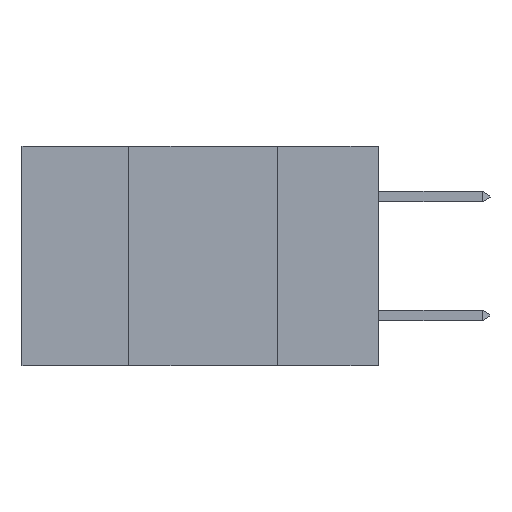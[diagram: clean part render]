
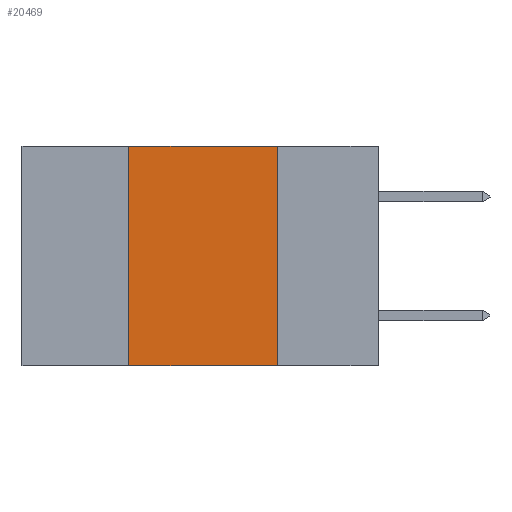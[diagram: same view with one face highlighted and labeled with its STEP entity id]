
A CAD part, left-side view. The second image highlights one B-rep face of the part: STEP entity #20469.
In plain terms, the highlighted planar face has unit normal (-1, 0, 0).
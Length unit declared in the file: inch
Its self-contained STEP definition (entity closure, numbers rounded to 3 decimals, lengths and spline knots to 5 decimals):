
#223 = CARTESIAN_POINT ( 'NONE',  ( 0., 0.6, -0.37 ) ) ;
#341 = DIRECTION ( 'NONE',  ( 0., 0., 1. ) ) ;
#450 = EDGE_CURVE ( 'NONE', #16474, #4178, #8391, .T. ) ;
#529 = ORIENTED_EDGE ( 'NONE', *, *, #15107, .F. ) ;
#792 = VERTEX_POINT ( 'NONE', #21328 ) ;
#1607 = CARTESIAN_POINT ( 'NONE',  ( 0., 0.6, 0. ) ) ;
#2045 = CARTESIAN_POINT ( 'NONE',  ( 0., 0.42, 0. ) ) ;
#2080 = LINE ( 'NONE', #223, #2353 ) ;
#2353 = VECTOR ( 'NONE', #6689, 39.37008 ) ;
#4178 = VERTEX_POINT ( 'NONE', #13958 ) ;
#5643 = VECTOR ( 'NONE', #8329, 39.37008 ) ;
#6024 = VECTOR ( 'NONE', #9877, 39.37008 ) ;
#6689 = DIRECTION ( 'NONE',  ( 0., -1., 0. ) ) ;
#8209 = ORIENTED_EDGE ( 'NONE', *, *, #450, .F. ) ;
#8329 = DIRECTION ( 'NONE',  ( 0., -1., 0. ) ) ;
#8335 = DIRECTION ( 'NONE',  ( 0., 0., -1. ) ) ;
#8364 = ORIENTED_EDGE ( 'NONE', *, *, #14026, .T. ) ;
#8391 = LINE ( 'NONE', #2045, #12371 ) ;
#8765 = FACE_OUTER_BOUND ( 'NONE', #16736, .T. ) ;
#8934 = LINE ( 'NONE', #11384, #6024 ) ;
#9877 = DIRECTION ( 'NONE',  ( 0., 0., -1. ) ) ;
#10109 = CARTESIAN_POINT ( 'NONE',  ( 0., 0.6, 0. ) ) ;
#11384 = CARTESIAN_POINT ( 'NONE',  ( 0., 0.17, 0. ) ) ;
#12371 = VECTOR ( 'NONE', #341, 39.37008 ) ;
#13013 = CARTESIAN_POINT ( 'NONE',  ( 0., 0.17, 0. ) ) ;
#13885 = AXIS2_PLACEMENT_3D ( 'NONE', #1607, #18480, #8335 ) ;
#13958 = CARTESIAN_POINT ( 'NONE',  ( 0., 0.42, 0. ) ) ;
#14026 = EDGE_CURVE ( 'NONE', #16474, #792, #2080, .T. ) ;
#14816 = CARTESIAN_POINT ( 'NONE',  ( 0., 0.42, -0.37 ) ) ;
#15107 = EDGE_CURVE ( 'NONE', #16400, #792, #8934, .T. ) ;
#16400 = VERTEX_POINT ( 'NONE', #13013 ) ;
#16474 = VERTEX_POINT ( 'NONE', #14816 ) ;
#16573 = PLANE ( 'NONE',  #13885 ) ;
#16736 = EDGE_LOOP ( 'NONE', ( #529, #18828, #8209, #8364 ) ) ;
#17124 = EDGE_CURVE ( 'NONE', #4178, #16400, #20902, .T. ) ;
#18480 = DIRECTION ( 'NONE',  ( 1., 0., 0. ) ) ;
#18828 = ORIENTED_EDGE ( 'NONE', *, *, #17124, .F. ) ;
#20469 = ADVANCED_FACE ( 'NONE', ( #8765 ), #16573, .F. ) ;
#20902 = LINE ( 'NONE', #10109, #5643 ) ;
#21328 = CARTESIAN_POINT ( 'NONE',  ( 0., 0.17, -0.37 ) ) ;
